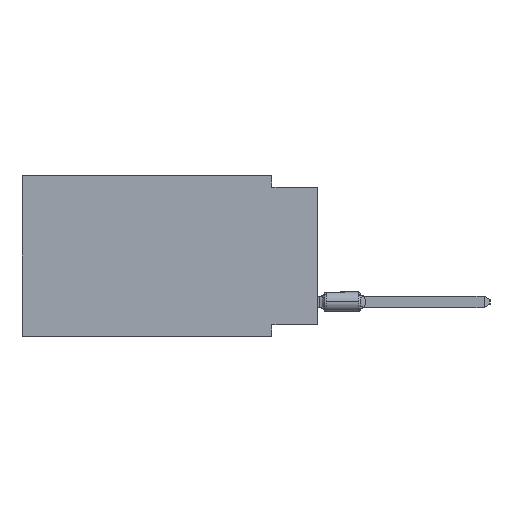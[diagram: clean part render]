
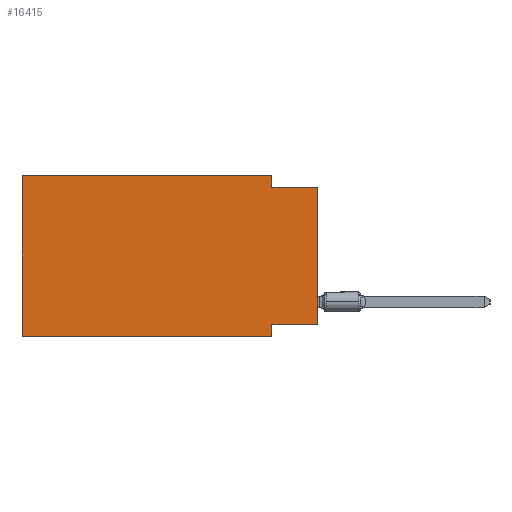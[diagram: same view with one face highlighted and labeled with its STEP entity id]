
A CAD part, left-side view. The second image highlights one B-rep face of the part: STEP entity #16415.
In plain terms, the highlighted planar face has unit normal (-1, 0, 0).
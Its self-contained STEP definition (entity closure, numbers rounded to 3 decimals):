
#1014 = CARTESIAN_POINT ( 'NONE',  ( 0., 16.383, -8.89 ) ) ;
#4595 = EDGE_CURVE ( 'NONE', #63687, #24152, #54428, .T. ) ;
#6011 = VECTOR ( 'NONE', #43356, 1000. ) ;
#7785 = PLANE ( 'NONE',  #45772 ) ;
#8842 = CARTESIAN_POINT ( 'NONE',  ( 0., 2.54, -0.635 ) ) ;
#12386 = CARTESIAN_POINT ( 'NONE',  ( 0., 16.383, 0. ) ) ;
#12531 = VECTOR ( 'NONE', #13505, 1000. ) ;
#12604 = EDGE_CURVE ( 'NONE', #67700, #31625, #47707, .T. ) ;
#13215 = VERTEX_POINT ( 'NONE', #64025 ) ;
#13397 = EDGE_CURVE ( 'NONE', #59083, #13215, #19149, .T. ) ;
#13505 = DIRECTION ( 'NONE',  ( 0., 0., 1. ) ) ;
#13615 = LINE ( 'NONE', #29717, #65126 ) ;
#14075 = VECTOR ( 'NONE', #66874, 1000. ) ;
#15498 = ORIENTED_EDGE ( 'NONE', *, *, #62500, .F. ) ;
#16415 = ADVANCED_FACE ( 'NONE', ( #35065 ), #7785, .F. ) ;
#18759 = LINE ( 'NONE', #40079, #12531 ) ;
#19149 = LINE ( 'NONE', #24748, #44547 ) ;
#19655 = DIRECTION ( 'NONE',  ( 1., 0., 0. ) ) ;
#20936 = VERTEX_POINT ( 'NONE', #50253 ) ;
#21358 = ORIENTED_EDGE ( 'NONE', *, *, #28441, .F. ) ;
#21586 = CARTESIAN_POINT ( 'NONE',  ( 0., 0., -0.635 ) ) ;
#23082 = LINE ( 'NONE', #32870, #6011 ) ;
#24152 = VERTEX_POINT ( 'NONE', #38018 ) ;
#24748 = CARTESIAN_POINT ( 'NONE',  ( 0., 16.383, -8.89 ) ) ;
#25506 = EDGE_CURVE ( 'NONE', #59083, #35702, #18759, .T. ) ;
#25619 = EDGE_LOOP ( 'NONE', ( #33809, #35099, #15498, #21358, #37943, #32436, #40035, #31635 ) ) ;
#28441 = EDGE_CURVE ( 'NONE', #35702, #20936, #13615, .T. ) ;
#29319 = DIRECTION ( 'NONE',  ( 0., -1., 0. ) ) ;
#29717 = CARTESIAN_POINT ( 'NONE',  ( 0., 16.383, 0. ) ) ;
#30060 = VECTOR ( 'NONE', #62080, 1000. ) ;
#30249 = CARTESIAN_POINT ( 'NONE',  ( 0., 0., -8.255 ) ) ;
#31625 = VERTEX_POINT ( 'NONE', #51986 ) ;
#31635 = ORIENTED_EDGE ( 'NONE', *, *, #12604, .F. ) ;
#32436 = ORIENTED_EDGE ( 'NONE', *, *, #13397, .T. ) ;
#32870 = CARTESIAN_POINT ( 'NONE',  ( 0., 2.54, 0. ) ) ;
#33809 = ORIENTED_EDGE ( 'NONE', *, *, #66024, .T. ) ;
#35065 = FACE_OUTER_BOUND ( 'NONE', #25619, .T. ) ;
#35099 = ORIENTED_EDGE ( 'NONE', *, *, #4595, .F. ) ;
#35529 = CARTESIAN_POINT ( 'NONE',  ( 0., 2.54, -8.89 ) ) ;
#35702 = VERTEX_POINT ( 'NONE', #12386 ) ;
#37943 = ORIENTED_EDGE ( 'NONE', *, *, #25506, .F. ) ;
#38018 = CARTESIAN_POINT ( 'NONE',  ( 0., 0., -0.635 ) ) ;
#39969 = EDGE_CURVE ( 'NONE', #31625, #13215, #46022, .T. ) ;
#40035 = ORIENTED_EDGE ( 'NONE', *, *, #39969, .F. ) ;
#40079 = CARTESIAN_POINT ( 'NONE',  ( 0., 16.383, 0. ) ) ;
#43356 = DIRECTION ( 'NONE',  ( 0., 0., -1. ) ) ;
#44452 = VECTOR ( 'NONE', #62729, 1000. ) ;
#44547 = VECTOR ( 'NONE', #29319, 1000. ) ;
#45551 = DIRECTION ( 'NONE',  ( 0., 0., -1. ) ) ;
#45772 = AXIS2_PLACEMENT_3D ( 'NONE', #51817, #19655, #45551 ) ;
#45911 = LINE ( 'NONE', #56075, #14075 ) ;
#46022 = LINE ( 'NONE', #35529, #30060 ) ;
#47707 = LINE ( 'NONE', #30249, #44452 ) ;
#50253 = CARTESIAN_POINT ( 'NONE',  ( 0., 2.54, 0. ) ) ;
#51025 = DIRECTION ( 'NONE',  ( 0., -1., 0. ) ) ;
#51817 = CARTESIAN_POINT ( 'NONE',  ( 0., 16.383, 0. ) ) ;
#51986 = CARTESIAN_POINT ( 'NONE',  ( 0., 2.54, -8.255 ) ) ;
#52825 = CARTESIAN_POINT ( 'NONE',  ( 0., 0., -8.255 ) ) ;
#54428 = LINE ( 'NONE', #21586, #63389 ) ;
#56075 = CARTESIAN_POINT ( 'NONE',  ( 0., 0., 0. ) ) ;
#59083 = VERTEX_POINT ( 'NONE', #1014 ) ;
#62080 = DIRECTION ( 'NONE',  ( 0., 0., -1. ) ) ;
#62500 = EDGE_CURVE ( 'NONE', #20936, #63687, #23082, .T. ) ;
#62729 = DIRECTION ( 'NONE',  ( 0., 1., 0. ) ) ;
#63389 = VECTOR ( 'NONE', #64198, 1000. ) ;
#63687 = VERTEX_POINT ( 'NONE', #8842 ) ;
#64025 = CARTESIAN_POINT ( 'NONE',  ( 0., 2.54, -8.89 ) ) ;
#64198 = DIRECTION ( 'NONE',  ( 0., -1., 0. ) ) ;
#65126 = VECTOR ( 'NONE', #51025, 1000. ) ;
#66024 = EDGE_CURVE ( 'NONE', #67700, #24152, #45911, .T. ) ;
#66874 = DIRECTION ( 'NONE',  ( 0., 0., 1. ) ) ;
#67700 = VERTEX_POINT ( 'NONE', #52825 ) ;
